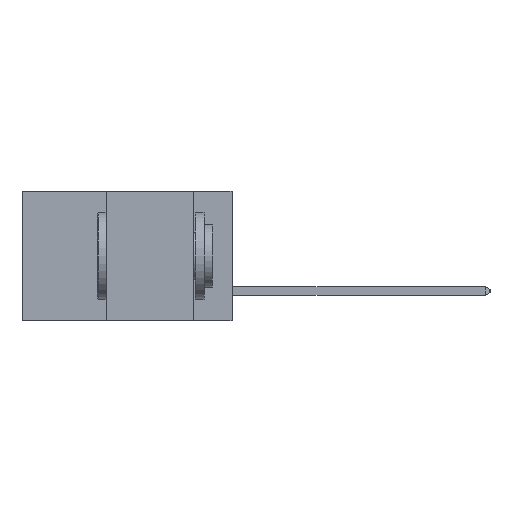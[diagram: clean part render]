
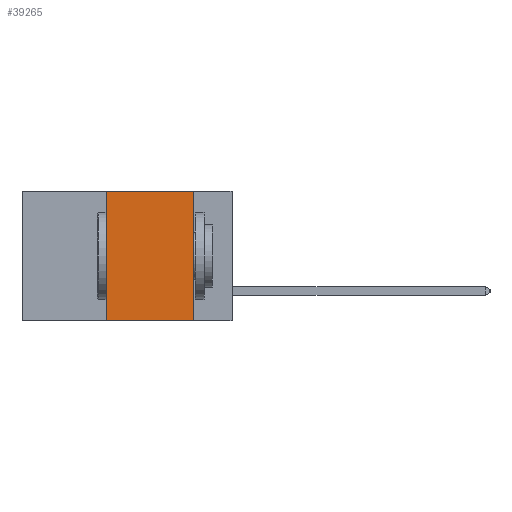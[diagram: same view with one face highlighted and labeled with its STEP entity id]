
A CAD part, left-side view. The second image highlights one B-rep face of the part: STEP entity #39265.
In plain terms, the highlighted planar face has unit normal (-1, 0, 0).
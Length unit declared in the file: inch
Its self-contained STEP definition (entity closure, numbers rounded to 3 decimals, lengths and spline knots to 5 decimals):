
#632 = LINE ( 'NONE', #1831, #39569 ) ;
#761 = VECTOR ( 'NONE', #37926, 39.37008 ) ;
#1831 = CARTESIAN_POINT ( 'NONE',  ( 0., 0.6, 0. ) ) ;
#1914 = VECTOR ( 'NONE', #17628, 39.37008 ) ;
#2065 = DIRECTION ( 'NONE',  ( 0., 0., -1. ) ) ;
#2581 = EDGE_CURVE ( 'NONE', #31896, #14677, #11203, .T. ) ;
#3630 = DIRECTION ( 'NONE',  ( 0., 0., 1. ) ) ;
#5008 = DIRECTION ( 'NONE',  ( 0., -1., 0. ) ) ;
#8832 = CARTESIAN_POINT ( 'NONE',  ( 0., 0.36, 0. ) ) ;
#10783 = LINE ( 'NONE', #12733, #34206 ) ;
#11203 = LINE ( 'NONE', #29812, #1914 ) ;
#12733 = CARTESIAN_POINT ( 'NONE',  ( 0., 0.36, 0. ) ) ;
#13284 = ORIENTED_EDGE ( 'NONE', *, *, #2581, .F. ) ;
#14677 = VERTEX_POINT ( 'NONE', #25371 ) ;
#17502 = CARTESIAN_POINT ( 'NONE',  ( 0., 0.6, 0. ) ) ;
#17628 = DIRECTION ( 'NONE',  ( 0., 0., -1. ) ) ;
#20599 = DIRECTION ( 'NONE',  ( 1., 0., 0. ) ) ;
#21570 = EDGE_CURVE ( 'NONE', #32007, #31896, #632, .T. ) ;
#23337 = ORIENTED_EDGE ( 'NONE', *, *, #32226, .F. ) ;
#23772 = EDGE_LOOP ( 'NONE', ( #13284, #24271, #23337, #37486 ) ) ;
#24271 = ORIENTED_EDGE ( 'NONE', *, *, #21570, .F. ) ;
#25371 = CARTESIAN_POINT ( 'NONE',  ( 0., 0.11, -0.37 ) ) ;
#25398 = LINE ( 'NONE', #31786, #761 ) ;
#29812 = CARTESIAN_POINT ( 'NONE',  ( 0., 0.11, 0. ) ) ;
#31254 = CARTESIAN_POINT ( 'NONE',  ( 0., 0.36, -0.37 ) ) ;
#31786 = CARTESIAN_POINT ( 'NONE',  ( 0., 0.6, -0.37 ) ) ;
#31896 = VERTEX_POINT ( 'NONE', #35855 ) ;
#32007 = VERTEX_POINT ( 'NONE', #8832 ) ;
#32226 = EDGE_CURVE ( 'NONE', #35421, #32007, #10783, .T. ) ;
#33409 = AXIS2_PLACEMENT_3D ( 'NONE', #17502, #20599, #2065 ) ;
#33862 = FACE_OUTER_BOUND ( 'NONE', #23772, .T. ) ;
#34206 = VECTOR ( 'NONE', #3630, 39.37008 ) ;
#35421 = VERTEX_POINT ( 'NONE', #31254 ) ;
#35803 = PLANE ( 'NONE',  #33409 ) ;
#35855 = CARTESIAN_POINT ( 'NONE',  ( 0., 0.11, 0. ) ) ;
#37486 = ORIENTED_EDGE ( 'NONE', *, *, #37841, .T. ) ;
#37841 = EDGE_CURVE ( 'NONE', #35421, #14677, #25398, .T. ) ;
#37926 = DIRECTION ( 'NONE',  ( 0., -1., 0. ) ) ;
#39265 = ADVANCED_FACE ( 'NONE', ( #33862 ), #35803, .F. ) ;
#39569 = VECTOR ( 'NONE', #5008, 39.37008 ) ;
